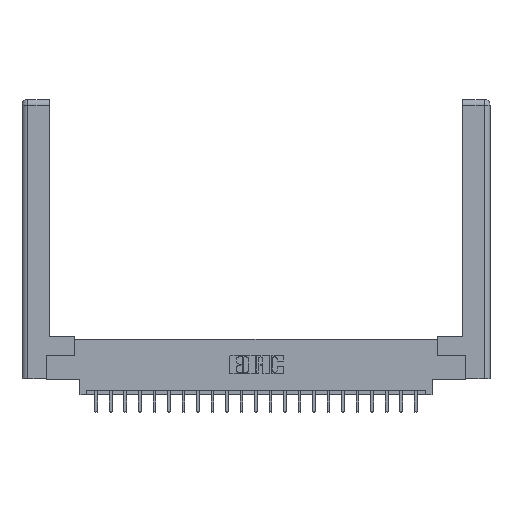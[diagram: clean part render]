
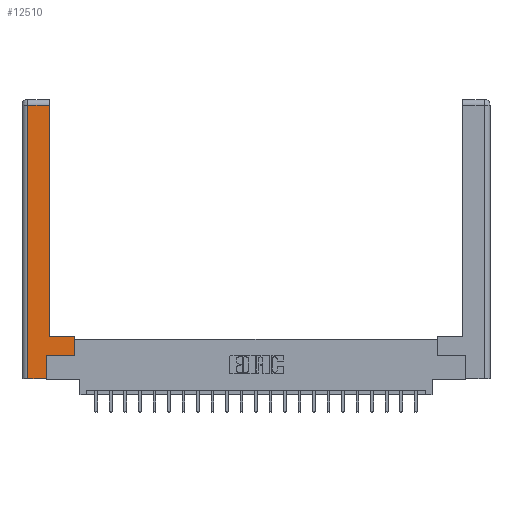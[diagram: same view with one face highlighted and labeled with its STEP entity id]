
A CAD part, top view. The second image highlights one B-rep face of the part: STEP entity #12510.
In plain terms, the highlighted planar face has unit normal (0, 0, 1).
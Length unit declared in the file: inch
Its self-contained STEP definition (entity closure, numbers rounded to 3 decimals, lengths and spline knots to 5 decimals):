
#62 = VECTOR ( 'NONE', #15573, 39.37008 ) ;
#532 = LINE ( 'NONE', #4382, #6149 ) ;
#565 = CARTESIAN_POINT ( 'NONE',  ( 0.265, 0.245, 0. ) ) ;
#1076 = EDGE_CURVE ( 'NONE', #9914, #11512, #8608, .T. ) ;
#1167 = LINE ( 'NONE', #2793, #19615 ) ;
#1192 = LINE ( 'NONE', #12117, #16294 ) ;
#1720 = CARTESIAN_POINT ( 'NONE',  ( 0.295, 3., 0. ) ) ;
#2298 = CARTESIAN_POINT ( 'NONE',  ( 0.295, 0.45, 0. ) ) ;
#2793 = CARTESIAN_POINT ( 'NONE',  ( 0.0615, 0., 0. ) ) ;
#2867 = VECTOR ( 'NONE', #8864, 39.37008 ) ;
#3586 = EDGE_CURVE ( 'NONE', #16752, #5325, #9528, .T. ) ;
#4382 = CARTESIAN_POINT ( 'NONE',  ( 0.295, 0.45, 0. ) ) ;
#4706 = EDGE_CURVE ( 'NONE', #8256, #16752, #19495, .T. ) ;
#5325 = VERTEX_POINT ( 'NONE', #565 ) ;
#5368 = CARTESIAN_POINT ( 'NONE',  ( 0.0615, 2.94, 0. ) ) ;
#5725 = LINE ( 'NONE', #12658, #2867 ) ;
#6149 = VECTOR ( 'NONE', #14799, 39.37008 ) ;
#6371 = CARTESIAN_POINT ( 'NONE',  ( 0.265, 0.245, 0. ) ) ;
#6447 = ORIENTED_EDGE ( 'NONE', *, *, #19222, .T. ) ;
#6819 = DIRECTION ( 'NONE',  ( 0., 0., -1. ) ) ;
#6918 = DIRECTION ( 'NONE',  ( 0., 1., 0. ) ) ;
#6983 = DIRECTION ( 'NONE',  ( -1., 0., 0. ) ) ;
#7109 = ORIENTED_EDGE ( 'NONE', *, *, #3586, .T. ) ;
#8252 = EDGE_CURVE ( 'NONE', #11512, #17252, #15432, .T. ) ;
#8256 = VERTEX_POINT ( 'NONE', #22871 ) ;
#8543 = EDGE_CURVE ( 'NONE', #17252, #8256, #1167, .T. ) ;
#8608 = LINE ( 'NONE', #1720, #13871 ) ;
#8864 = DIRECTION ( 'NONE',  ( 1., 0., 0. ) ) ;
#9027 = ORIENTED_EDGE ( 'NONE', *, *, #10229, .T. ) ;
#9528 = LINE ( 'NONE', #6371, #14804 ) ;
#9847 = DIRECTION ( 'NONE',  ( 1., 0., 0. ) ) ;
#9914 = VERTEX_POINT ( 'NONE', #2298 ) ;
#10229 = EDGE_CURVE ( 'NONE', #5325, #10265, #5725, .T. ) ;
#10265 = VERTEX_POINT ( 'NONE', #15935 ) ;
#10543 = CARTESIAN_POINT ( 'NONE',  ( 0.0615, 2.94, 0. ) ) ;
#11420 = ORIENTED_EDGE ( 'NONE', *, *, #4706, .T. ) ;
#11512 = VERTEX_POINT ( 'NONE', #21992 ) ;
#12117 = CARTESIAN_POINT ( 'NONE',  ( 0.565, 0.45, 0. ) ) ;
#12510 = ADVANCED_FACE ( 'NONE', ( #22386 ), #14190, .F. ) ;
#12658 = CARTESIAN_POINT ( 'NONE',  ( 0.565, 0.245, 0. ) ) ;
#13193 = ORIENTED_EDGE ( 'NONE', *, *, #1076, .T. ) ;
#13648 = DIRECTION ( 'NONE',  ( 0., -1., 0. ) ) ;
#13871 = VECTOR ( 'NONE', #6918, 39.37008 ) ;
#13904 = VECTOR ( 'NONE', #9847, 39.37008 ) ;
#14190 = PLANE ( 'NONE',  #21371 ) ;
#14282 = VERTEX_POINT ( 'NONE', #15332 ) ;
#14799 = DIRECTION ( 'NONE',  ( -1., 0., 0. ) ) ;
#14804 = VECTOR ( 'NONE', #20603, 39.37008 ) ;
#15332 = CARTESIAN_POINT ( 'NONE',  ( 0.565, 0.45, 0. ) ) ;
#15432 = LINE ( 'NONE', #10543, #62 ) ;
#15573 = DIRECTION ( 'NONE',  ( -1., 0., 0. ) ) ;
#15935 = CARTESIAN_POINT ( 'NONE',  ( 0.565, 0.245, 0. ) ) ;
#16146 = EDGE_CURVE ( 'NONE', #10265, #14282, #1192, .T. ) ;
#16294 = VECTOR ( 'NONE', #17361, 39.37008 ) ;
#16752 = VERTEX_POINT ( 'NONE', #23195 ) ;
#17252 = VERTEX_POINT ( 'NONE', #5368 ) ;
#17361 = DIRECTION ( 'NONE',  ( 0., 1., 0. ) ) ;
#17482 = CARTESIAN_POINT ( 'NONE',  ( 0., 0., 0. ) ) ;
#18269 = EDGE_LOOP ( 'NONE', ( #13193, #22589, #21825, #11420, #7109, #9027, #20220, #6447 ) ) ;
#18656 = CARTESIAN_POINT ( 'NONE',  ( 0.265, 0., 0. ) ) ;
#19222 = EDGE_CURVE ( 'NONE', #14282, #9914, #532, .T. ) ;
#19495 = LINE ( 'NONE', #18656, #13904 ) ;
#19615 = VECTOR ( 'NONE', #13648, 39.37008 ) ;
#20220 = ORIENTED_EDGE ( 'NONE', *, *, #16146, .T. ) ;
#20603 = DIRECTION ( 'NONE',  ( 0., 1., 0. ) ) ;
#21371 = AXIS2_PLACEMENT_3D ( 'NONE', #17482, #6819, #6983 ) ;
#21825 = ORIENTED_EDGE ( 'NONE', *, *, #8543, .T. ) ;
#21992 = CARTESIAN_POINT ( 'NONE',  ( 0.295, 2.94, 0. ) ) ;
#22386 = FACE_OUTER_BOUND ( 'NONE', #18269, .T. ) ;
#22589 = ORIENTED_EDGE ( 'NONE', *, *, #8252, .T. ) ;
#22871 = CARTESIAN_POINT ( 'NONE',  ( 0.0615, 0., 0. ) ) ;
#23195 = CARTESIAN_POINT ( 'NONE',  ( 0.265, 0., 0. ) ) ;
